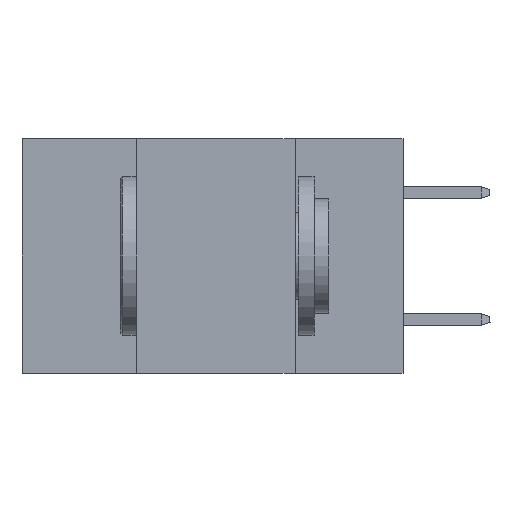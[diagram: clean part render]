
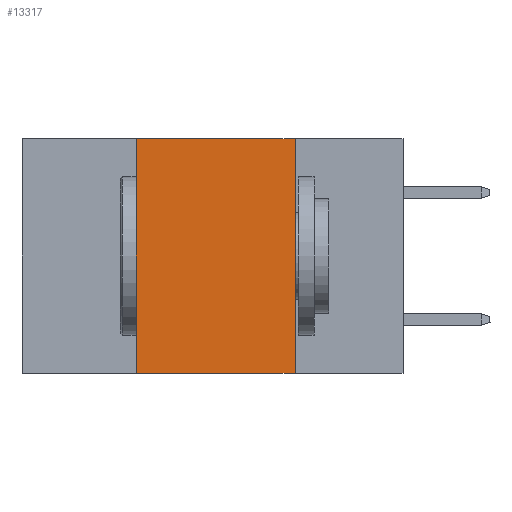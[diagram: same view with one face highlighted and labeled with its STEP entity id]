
A CAD part, left-side view. The second image highlights one B-rep face of the part: STEP entity #13317.
In plain terms, the highlighted planar face has unit normal (-1, 0, 0).
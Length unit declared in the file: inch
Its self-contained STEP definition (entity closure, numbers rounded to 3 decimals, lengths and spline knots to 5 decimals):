
#258 = CARTESIAN_POINT ( 'NONE',  ( 0., 0.42, -0.37 ) ) ;
#312 = CARTESIAN_POINT ( 'NONE',  ( 0., 0.6, 0. ) ) ;
#776 = EDGE_CURVE ( 'NONE', #11629, #6233, #9793, .T. ) ;
#1300 = CARTESIAN_POINT ( 'NONE',  ( 0., 0.17, -0.37 ) ) ;
#2455 = DIRECTION ( 'NONE',  ( 1., 0., 0. ) ) ;
#2720 = LINE ( 'NONE', #7118, #3669 ) ;
#3669 = VECTOR ( 'NONE', #11530, 39.37008 ) ;
#3734 = PLANE ( 'NONE',  #4115 ) ;
#4115 = AXIS2_PLACEMENT_3D ( 'NONE', #312, #2455, #9294 ) ;
#4518 = CARTESIAN_POINT ( 'NONE',  ( 0., 0.17, 0. ) ) ;
#5628 = LINE ( 'NONE', #4518, #9482 ) ;
#6233 = VERTEX_POINT ( 'NONE', #14178 ) ;
#6338 = EDGE_CURVE ( 'NONE', #6233, #7449, #2720, .T. ) ;
#6431 = CARTESIAN_POINT ( 'NONE',  ( 0., 0.17, 0. ) ) ;
#6560 = DIRECTION ( 'NONE',  ( 0., 0., 1. ) ) ;
#6989 = CARTESIAN_POINT ( 'NONE',  ( 0., 0.6, -0.37 ) ) ;
#7118 = CARTESIAN_POINT ( 'NONE',  ( 0., 0.6, 0. ) ) ;
#7449 = VERTEX_POINT ( 'NONE', #6431 ) ;
#8062 = EDGE_CURVE ( 'NONE', #7449, #11601, #5628, .T. ) ;
#8140 = ORIENTED_EDGE ( 'NONE', *, *, #776, .F. ) ;
#8695 = ORIENTED_EDGE ( 'NONE', *, *, #8062, .F. ) ;
#8931 = DIRECTION ( 'NONE',  ( 0., 0., -1. ) ) ;
#9088 = DIRECTION ( 'NONE',  ( 0., -1., 0. ) ) ;
#9294 = DIRECTION ( 'NONE',  ( 0., 0., -1. ) ) ;
#9482 = VECTOR ( 'NONE', #8931, 39.37008 ) ;
#9793 = LINE ( 'NONE', #13056, #11750 ) ;
#9887 = VECTOR ( 'NONE', #9088, 39.37008 ) ;
#10230 = LINE ( 'NONE', #6989, #9887 ) ;
#11530 = DIRECTION ( 'NONE',  ( 0., -1., 0. ) ) ;
#11601 = VERTEX_POINT ( 'NONE', #1300 ) ;
#11629 = VERTEX_POINT ( 'NONE', #258 ) ;
#11750 = VECTOR ( 'NONE', #6560, 39.37008 ) ;
#11945 = EDGE_LOOP ( 'NONE', ( #8695, #12266, #8140, #13757 ) ) ;
#12266 = ORIENTED_EDGE ( 'NONE', *, *, #6338, .F. ) ;
#13056 = CARTESIAN_POINT ( 'NONE',  ( 0., 0.42, 0. ) ) ;
#13308 = EDGE_CURVE ( 'NONE', #11629, #11601, #10230, .T. ) ;
#13317 = ADVANCED_FACE ( 'NONE', ( #13511 ), #3734, .F. ) ;
#13511 = FACE_OUTER_BOUND ( 'NONE', #11945, .T. ) ;
#13757 = ORIENTED_EDGE ( 'NONE', *, *, #13308, .T. ) ;
#14178 = CARTESIAN_POINT ( 'NONE',  ( 0., 0.42, 0. ) ) ;
